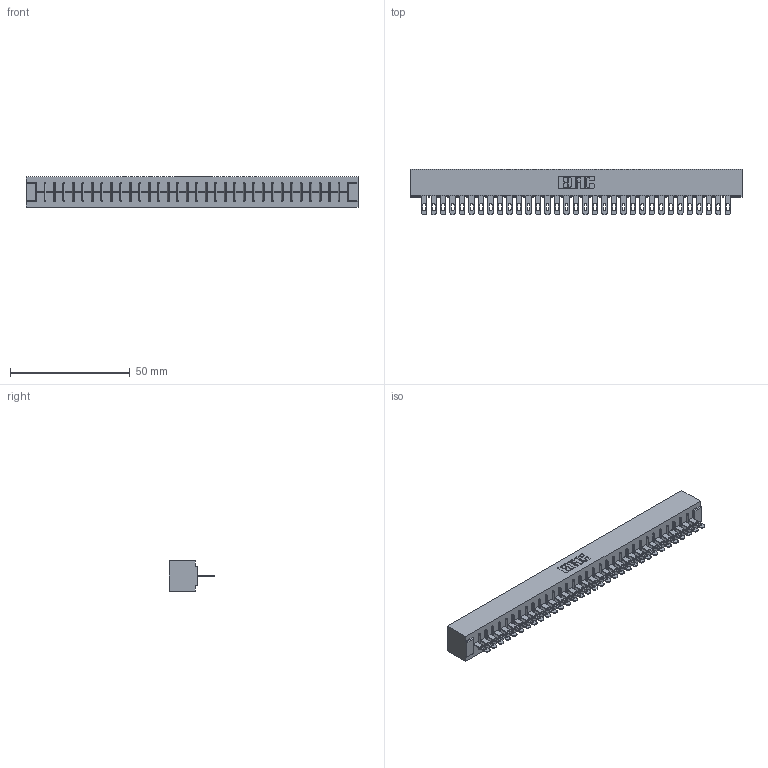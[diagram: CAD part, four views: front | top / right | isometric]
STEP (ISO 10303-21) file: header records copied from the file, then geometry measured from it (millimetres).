
FILE_DESCRIPTION (( 'STEP AP203' ), '1' );
FILE_NAME ('316-033-500-101.STEP', '2018-07-31T03:47:18', ( '' ), ( '' ), 'SwSTEP 2.0', 'SolidWorks 2016', '' );
FILE_SCHEMA (( 'CONFIG_CONTROL_DESIGN' ));
Length unit declared in the file: inch
Products named in the file (3): 306 Part_No Mounting; 306-290-001_100; 316-033-500-101
Assembly tree (34 placements, depth 2):
  316-033-500-101
    306 Part_No Mounting
    306-290-001_100  x33
Bounding box: 138.63 x 18.87 x 12.7 mm (x, y, z)
Volume: 15940.8 mm3; surface area: 16975.4 mm2
Topology: 34 solids, 34 shells, 2616 faces, 7387 edges, 4746 vertices
Faces by surface type: plane 1714, cylinder 770, sphere 132
Entity records: 31826 total; most frequent: CARTESIAN_POINT 5342, ORIENTED_EDGE 5294, DIRECTION 5269, EDGE_CURVE 2647, VECTOR 2067, LINE 2067, VERTEX_POINT 1674, AXIS2_PLACEMENT_3D 1601
